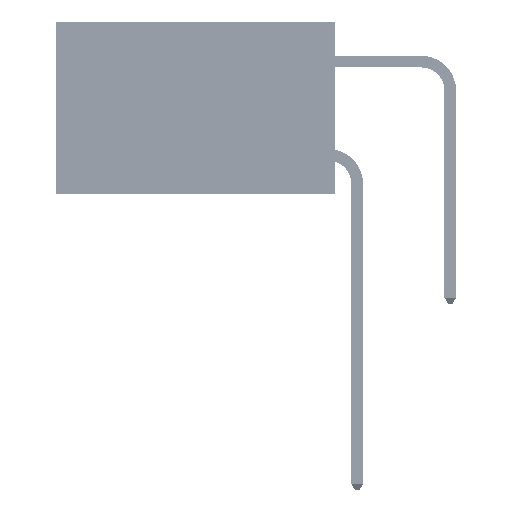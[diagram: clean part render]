
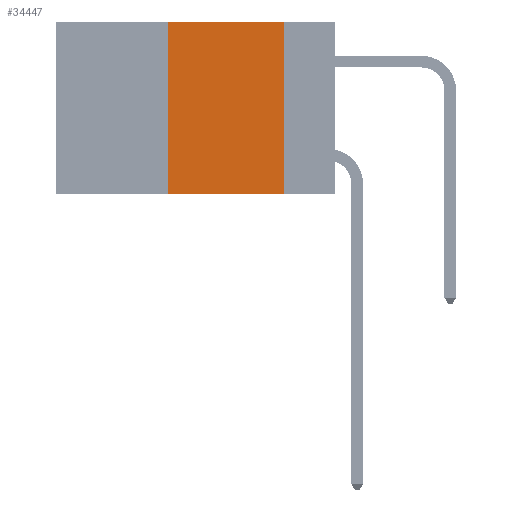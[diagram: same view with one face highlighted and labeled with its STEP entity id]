
A CAD part, left-side view. The second image highlights one B-rep face of the part: STEP entity #34447.
In plain terms, the highlighted planar face has unit normal (-1, 0, 0).
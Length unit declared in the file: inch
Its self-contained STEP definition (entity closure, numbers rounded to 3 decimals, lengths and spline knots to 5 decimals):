
#343 = DIRECTION ( 'NONE',  ( 0., -1., 0. ) ) ;
#1661 = VECTOR ( 'NONE', #36511, 39.37008 ) ;
#1979 = EDGE_CURVE ( 'NONE', #6830, #44337, #29185, .T. ) ;
#2304 = CARTESIAN_POINT ( 'NONE',  ( 0., 0.11, 0. ) ) ;
#2868 = AXIS2_PLACEMENT_3D ( 'NONE', #36248, #13930, #40043 ) ;
#6497 = CARTESIAN_POINT ( 'NONE',  ( 0., 0.36, 0. ) ) ;
#6697 = CARTESIAN_POINT ( 'NONE',  ( 0., 0.36, 0. ) ) ;
#6830 = VERTEX_POINT ( 'NONE', #8899 ) ;
#7848 = CARTESIAN_POINT ( 'NONE',  ( 0., 0.6, 0. ) ) ;
#8899 = CARTESIAN_POINT ( 'NONE',  ( 0., 0.36, -0.37 ) ) ;
#11165 = EDGE_CURVE ( 'NONE', #20627, #31771, #42828, .T. ) ;
#13930 = DIRECTION ( 'NONE',  ( 1., 0., 0. ) ) ;
#14574 = ORIENTED_EDGE ( 'NONE', *, *, #22037, .F. ) ;
#20555 = DIRECTION ( 'NONE',  ( 0., 0., -1. ) ) ;
#20627 = VERTEX_POINT ( 'NONE', #6497 ) ;
#22037 = EDGE_CURVE ( 'NONE', #6830, #20627, #31440, .T. ) ;
#23681 = EDGE_LOOP ( 'NONE', ( #30794, #36048, #14574, #46077 ) ) ;
#24136 = CARTESIAN_POINT ( 'NONE',  ( 0., 0.11, 0. ) ) ;
#26520 = CARTESIAN_POINT ( 'NONE',  ( 0., 0.11, -0.37 ) ) ;
#28787 = PLANE ( 'NONE',  #2868 ) ;
#29185 = LINE ( 'NONE', #29990, #47831 ) ;
#29462 = LINE ( 'NONE', #24136, #46947 ) ;
#29990 = CARTESIAN_POINT ( 'NONE',  ( 0., 0.6, -0.37 ) ) ;
#30794 = ORIENTED_EDGE ( 'NONE', *, *, #47925, .F. ) ;
#30866 = FACE_OUTER_BOUND ( 'NONE', #23681, .T. ) ;
#31440 = LINE ( 'NONE', #6697, #1661 ) ;
#31771 = VERTEX_POINT ( 'NONE', #2304 ) ;
#33581 = DIRECTION ( 'NONE',  ( 0., -1., 0. ) ) ;
#34447 = ADVANCED_FACE ( 'NONE', ( #30866 ), #28787, .F. ) ;
#36048 = ORIENTED_EDGE ( 'NONE', *, *, #11165, .F. ) ;
#36248 = CARTESIAN_POINT ( 'NONE',  ( 0., 0.6, 0. ) ) ;
#36511 = DIRECTION ( 'NONE',  ( 0., 0., 1. ) ) ;
#40043 = DIRECTION ( 'NONE',  ( 0., 0., -1. ) ) ;
#42828 = LINE ( 'NONE', #7848, #43984 ) ;
#43984 = VECTOR ( 'NONE', #343, 39.37008 ) ;
#44337 = VERTEX_POINT ( 'NONE', #26520 ) ;
#46077 = ORIENTED_EDGE ( 'NONE', *, *, #1979, .T. ) ;
#46947 = VECTOR ( 'NONE', #20555, 39.37008 ) ;
#47831 = VECTOR ( 'NONE', #33581, 39.37008 ) ;
#47925 = EDGE_CURVE ( 'NONE', #31771, #44337, #29462, .T. ) ;
